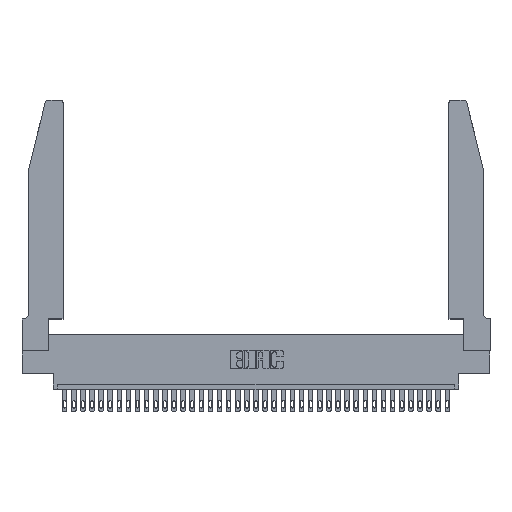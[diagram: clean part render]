
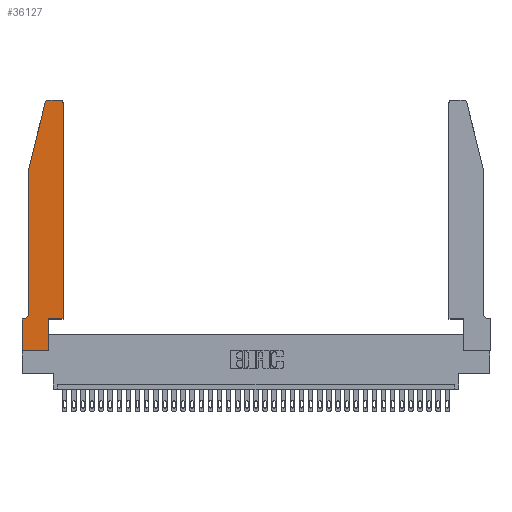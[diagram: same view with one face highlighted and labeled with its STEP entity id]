
A CAD part, top view. The second image highlights one B-rep face of the part: STEP entity #36127.
In plain terms, the highlighted planar face has unit normal (0, 0, 1).
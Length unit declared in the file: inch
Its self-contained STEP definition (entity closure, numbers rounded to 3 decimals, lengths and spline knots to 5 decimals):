
#83 = VERTEX_POINT ( 'NONE', #1605 ) ;
#279 = ORIENTED_EDGE ( 'NONE', *, *, #14043, .T. ) ;
#596 = CARTESIAN_POINT ( 'NONE',  ( 0.4505, 2.72, 0.37 ) ) ;
#999 = EDGE_CURVE ( 'NONE', #34435, #83, #36143, .T. ) ;
#1581 = ORIENTED_EDGE ( 'NONE', *, *, #35291, .T. ) ;
#1605 = CARTESIAN_POINT ( 'NONE',  ( 0.4505, 0.35, 0.37 ) ) ;
#1627 = EDGE_CURVE ( 'NONE', #28276, #34435, #30756, .T. ) ;
#1711 = CARTESIAN_POINT ( 'NONE',  ( 0.284, 2.75, 0.37 ) ) ;
#2120 = LINE ( 'NONE', #26740, #9657 ) ;
#2516 = CARTESIAN_POINT ( 'NONE',  ( 0., 0., 0.37 ) ) ;
#2915 = CARTESIAN_POINT ( 'NONE',  ( 0.2865, 0.35, 0.37 ) ) ;
#3022 = VECTOR ( 'NONE', #28064, 39.37008 ) ;
#3044 = CARTESIAN_POINT ( 'NONE',  ( 0., 0.35, 0.37 ) ) ;
#3403 = ORIENTED_EDGE ( 'NONE', *, *, #23423, .T. ) ;
#3651 = CARTESIAN_POINT ( 'NONE',  ( 0.2865, 0., 0.37 ) ) ;
#4320 = VERTEX_POINT ( 'NONE', #28821 ) ;
#4444 = VERTEX_POINT ( 'NONE', #34464 ) ;
#4456 = LINE ( 'NONE', #32930, #11542 ) ;
#5158 = ORIENTED_EDGE ( 'NONE', *, *, #24317, .T. ) ;
#5804 = DIRECTION ( 'NONE',  ( 1., 0., 0. ) ) ;
#5835 = VERTEX_POINT ( 'NONE', #3044 ) ;
#6390 = AXIS2_PLACEMENT_3D ( 'NONE', #13592, #29177, #31793 ) ;
#6991 = EDGE_CURVE ( 'NONE', #16478, #28276, #4456, .T. ) ;
#7013 = ORIENTED_EDGE ( 'NONE', *, *, #999, .T. ) ;
#8077 = CIRCLE ( 'NONE', #6390, 0.07 ) ;
#8239 = LINE ( 'NONE', #33761, #32757 ) ;
#8285 = EDGE_CURVE ( 'NONE', #5835, #16478, #2120, .T. ) ;
#8310 = VERTEX_POINT ( 'NONE', #35405 ) ;
#8786 = CARTESIAN_POINT ( 'NONE',  ( 0., 0.35, 0.37 ) ) ;
#9393 = CARTESIAN_POINT ( 'NONE',  ( 0.0055, 0.35, 0.37 ) ) ;
#9508 = EDGE_CURVE ( 'NONE', #16349, #5835, #8239, .T. ) ;
#9657 = VECTOR ( 'NONE', #32847, 39.37008 ) ;
#11041 = DIRECTION ( 'NONE',  ( -1., 0., 0. ) ) ;
#11073 = VECTOR ( 'NONE', #29959, 39.37008 ) ;
#11276 = VECTOR ( 'NONE', #19038, 39.37008 ) ;
#11414 = DIRECTION ( 'NONE',  ( 0., 0., 1. ) ) ;
#11542 = VECTOR ( 'NONE', #21675, 39.37008 ) ;
#12902 = ORIENTED_EDGE ( 'NONE', *, *, #9508, .T. ) ;
#13295 = DIRECTION ( 'NONE',  ( 1., 0., 0. ) ) ;
#13592 = CARTESIAN_POINT ( 'NONE',  ( 0.0055, 0.42, 0.37 ) ) ;
#13671 = CIRCLE ( 'NONE', #29033, 0.03 ) ;
#14043 = EDGE_CURVE ( 'NONE', #31270, #4444, #13671, .T. ) ;
#14812 = CARTESIAN_POINT ( 'NONE',  ( 0.2605, 2.75, 0.37 ) ) ;
#16349 = VERTEX_POINT ( 'NONE', #9393 ) ;
#16418 = DIRECTION ( 'NONE',  ( 0., 0., 1. ) ) ;
#16478 = VERTEX_POINT ( 'NONE', #2516 ) ;
#17539 = DIRECTION ( 'NONE',  ( 1., 0., 0. ) ) ;
#17966 = LINE ( 'NONE', #30550, #11276 ) ;
#19038 = DIRECTION ( 'NONE',  ( 0., 1., 0. ) ) ;
#20354 = PLANE ( 'NONE',  #21377 ) ;
#20837 = VECTOR ( 'NONE', #17539, 39.37008 ) ;
#21377 = AXIS2_PLACEMENT_3D ( 'NONE', #8786, #11414, #5804 ) ;
#21586 = CARTESIAN_POINT ( 'NONE',  ( 0.0755, 2., 0.37 ) ) ;
#21675 = DIRECTION ( 'NONE',  ( 1., 0., 0. ) ) ;
#22254 = CARTESIAN_POINT ( 'NONE',  ( 0.0755, 2., 0.37 ) ) ;
#22347 = LINE ( 'NONE', #21586, #30394 ) ;
#22369 = ORIENTED_EDGE ( 'NONE', *, *, #1627, .T. ) ;
#22691 = VERTEX_POINT ( 'NONE', #1711 ) ;
#22701 = FACE_OUTER_BOUND ( 'NONE', #35308, .T. ) ;
#22977 = EDGE_CURVE ( 'NONE', #4320, #25180, #25518, .T. ) ;
#23423 = EDGE_CURVE ( 'NONE', #25180, #16349, #8077, .T. ) ;
#23696 = VECTOR ( 'NONE', #30897, 39.37008 ) ;
#24109 = ORIENTED_EDGE ( 'NONE', *, *, #6991, .T. ) ;
#24168 = CARTESIAN_POINT ( 'NONE',  ( 0.4505, 0.35, 0.37 ) ) ;
#24187 = EDGE_CURVE ( 'NONE', #22691, #8310, #28106, .T. ) ;
#24317 = EDGE_CURVE ( 'NONE', #4444, #22691, #33849, .T. ) ;
#24554 = ORIENTED_EDGE ( 'NONE', *, *, #22977, .T. ) ;
#25180 = VERTEX_POINT ( 'NONE', #32918 ) ;
#25518 = LINE ( 'NONE', #22254, #23696 ) ;
#26186 = AXIS2_PLACEMENT_3D ( 'NONE', #33455, #33832, #30727 ) ;
#26740 = CARTESIAN_POINT ( 'NONE',  ( 0., 0., 0.37 ) ) ;
#26859 = ORIENTED_EDGE ( 'NONE', *, *, #24187, .T. ) ;
#27083 = DIRECTION ( 'NONE',  ( -0.239, -0.971, 0. ) ) ;
#27358 = ORIENTED_EDGE ( 'NONE', *, *, #8285, .T. ) ;
#28064 = DIRECTION ( 'NONE',  ( -1., 0., 0. ) ) ;
#28106 = CIRCLE ( 'NONE', #26186, 0.03 ) ;
#28276 = VERTEX_POINT ( 'NONE', #3651 ) ;
#28821 = CARTESIAN_POINT ( 'NONE',  ( 0.0755, 2., 0.37 ) ) ;
#29033 = AXIS2_PLACEMENT_3D ( 'NONE', #33533, #16418, #13295 ) ;
#29177 = DIRECTION ( 'NONE',  ( 0., 0., -1. ) ) ;
#29695 = CARTESIAN_POINT ( 'NONE',  ( 0.2865, 0.35, 0.37 ) ) ;
#29959 = DIRECTION ( 'NONE',  ( 0., 1., 0. ) ) ;
#30394 = VECTOR ( 'NONE', #27083, 39.37008 ) ;
#30550 = CARTESIAN_POINT ( 'NONE',  ( 0.4505, 0.35, 0.37 ) ) ;
#30727 = DIRECTION ( 'NONE',  ( 1., 0., 0. ) ) ;
#30756 = LINE ( 'NONE', #29695, #11073 ) ;
#30897 = DIRECTION ( 'NONE',  ( 0., -1., 0. ) ) ;
#31270 = VERTEX_POINT ( 'NONE', #596 ) ;
#31793 = DIRECTION ( 'NONE',  ( -1., 0., 0. ) ) ;
#32757 = VECTOR ( 'NONE', #11041, 39.37008 ) ;
#32847 = DIRECTION ( 'NONE',  ( 0., -1., 0. ) ) ;
#32918 = CARTESIAN_POINT ( 'NONE',  ( 0.0755, 0.42, 0.37 ) ) ;
#32930 = CARTESIAN_POINT ( 'NONE',  ( 0., 0., 0.37 ) ) ;
#33098 = ORIENTED_EDGE ( 'NONE', *, *, #34089, .T. ) ;
#33455 = CARTESIAN_POINT ( 'NONE',  ( 0.284, 2.72, 0.37 ) ) ;
#33533 = CARTESIAN_POINT ( 'NONE',  ( 0.4205, 2.72, 0.37 ) ) ;
#33761 = CARTESIAN_POINT ( 'NONE',  ( 0.0755, 0.35, 0.37 ) ) ;
#33832 = DIRECTION ( 'NONE',  ( 0., 0., 1. ) ) ;
#33849 = LINE ( 'NONE', #14812, #3022 ) ;
#34089 = EDGE_CURVE ( 'NONE', #83, #31270, #17966, .T. ) ;
#34435 = VERTEX_POINT ( 'NONE', #2915 ) ;
#34464 = CARTESIAN_POINT ( 'NONE',  ( 0.4205, 2.75, 0.37 ) ) ;
#35291 = EDGE_CURVE ( 'NONE', #8310, #4320, #22347, .T. ) ;
#35308 = EDGE_LOOP ( 'NONE', ( #5158, #26859, #1581, #24554, #3403, #12902, #27358, #24109, #22369, #7013, #33098, #279 ) ) ;
#35405 = CARTESIAN_POINT ( 'NONE',  ( 0.25487, 2.72718, 0.37 ) ) ;
#36127 = ADVANCED_FACE ( 'NONE', ( #22701 ), #20354, .T. ) ;
#36143 = LINE ( 'NONE', #24168, #20837 ) ;
